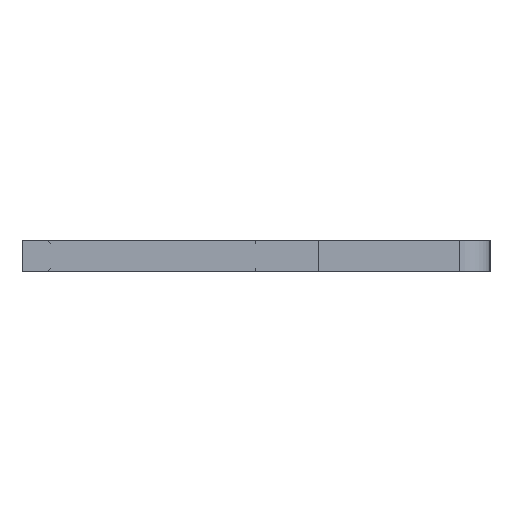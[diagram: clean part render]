
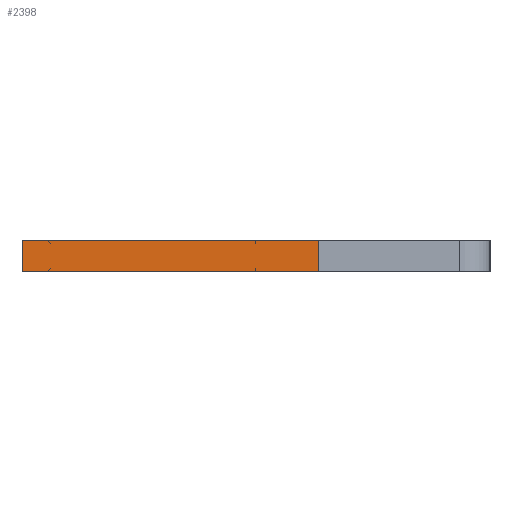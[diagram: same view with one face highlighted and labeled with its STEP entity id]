
A CAD part, left-side view. The second image highlights one B-rep face of the part: STEP entity #2398.
In plain terms, the highlighted face is planar.
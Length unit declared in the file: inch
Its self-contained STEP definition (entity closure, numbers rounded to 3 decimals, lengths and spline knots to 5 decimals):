
#25 = EDGE_CURVE ( 'NONE', #26, #1028, #1244, .T. ) ;
#26 = VERTEX_POINT ( 'NONE', #1856 ) ;
#71 = DIRECTION ( 'NONE',  ( 1., 0., 0. ) ) ;
#168 = EDGE_CURVE ( 'NONE', #2119, #683, #2328, .T. ) ;
#200 = DIRECTION ( 'NONE',  ( -1., 0., 0. ) ) ;
#225 = CARTESIAN_POINT ( 'NONE',  ( 0.01, -0.04, -0.04 ) ) ;
#347 = ORIENTED_EDGE ( 'NONE', *, *, #25, .T. ) ;
#385 = VECTOR ( 'NONE', #1549, 39.37008 ) ;
#491 = PLANE ( 'NONE',  #2700 ) ;
#656 = CARTESIAN_POINT ( 'NONE',  ( 0.01, 0.15, -0.04 ) ) ;
#683 = VERTEX_POINT ( 'NONE', #1876 ) ;
#1028 = VERTEX_POINT ( 'NONE', #2185 ) ;
#1068 = ORIENTED_EDGE ( 'NONE', *, *, #168, .F. ) ;
#1206 = EDGE_LOOP ( 'NONE', ( #1503, #1068, #2516, #347 ) ) ;
#1239 = EDGE_CURVE ( 'NONE', #26, #2119, #2493, .T. ) ;
#1244 = LINE ( 'NONE', #225, #1967 ) ;
#1431 = CARTESIAN_POINT ( 'NONE',  ( 0.01, 0.15, -0.04 ) ) ;
#1503 = ORIENTED_EDGE ( 'NONE', *, *, #2606, .T. ) ;
#1549 = DIRECTION ( 'NONE',  ( 0., 1., 0. ) ) ;
#1582 = DIRECTION ( 'NONE',  ( -1., 0., 0. ) ) ;
#1856 = CARTESIAN_POINT ( 'NONE',  ( 0.01, -0.04, -0.04 ) ) ;
#1876 = CARTESIAN_POINT ( 'NONE',  ( -0.01, 0.15, -0.04 ) ) ;
#1967 = VECTOR ( 'NONE', #200, 39.37008 ) ;
#2119 = VERTEX_POINT ( 'NONE', #656 ) ;
#2140 = CARTESIAN_POINT ( 'NONE',  ( 0.01, 0.15, -0.04 ) ) ;
#2185 = CARTESIAN_POINT ( 'NONE',  ( -0.01, -0.04, -0.04 ) ) ;
#2328 = LINE ( 'NONE', #2140, #2887 ) ;
#2398 = ADVANCED_FACE ( 'NONE', ( #3270 ), #491, .F. ) ;
#2417 = DIRECTION ( 'NONE',  ( 0., 1., 0. ) ) ;
#2493 = LINE ( 'NONE', #2983, #2759 ) ;
#2516 = ORIENTED_EDGE ( 'NONE', *, *, #1239, .F. ) ;
#2606 = EDGE_CURVE ( 'NONE', #1028, #683, #3393, .T. ) ;
#2700 = AXIS2_PLACEMENT_3D ( 'NONE', #1431, #3320, #71 ) ;
#2759 = VECTOR ( 'NONE', #2417, 39.37008 ) ;
#2887 = VECTOR ( 'NONE', #1582, 39.37008 ) ;
#2900 = CARTESIAN_POINT ( 'NONE',  ( -0.01, 0.15, -0.04 ) ) ;
#2983 = CARTESIAN_POINT ( 'NONE',  ( 0.01, 0.15, -0.04 ) ) ;
#3270 = FACE_OUTER_BOUND ( 'NONE', #1206, .T. ) ;
#3320 = DIRECTION ( 'NONE',  ( 0., 0., 1. ) ) ;
#3393 = LINE ( 'NONE', #2900, #385 ) ;
